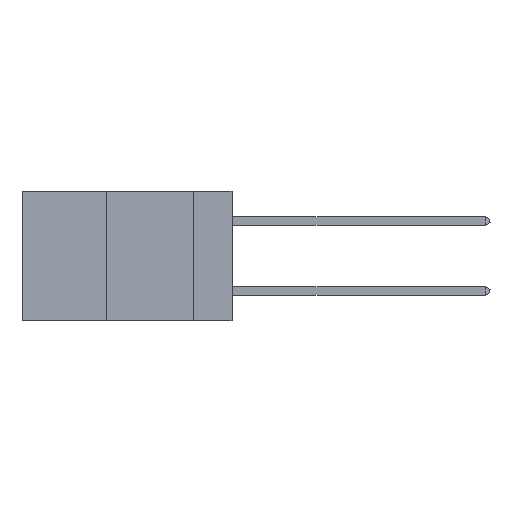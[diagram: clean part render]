
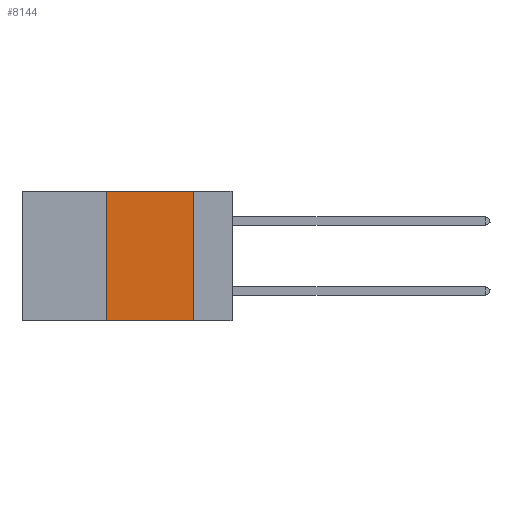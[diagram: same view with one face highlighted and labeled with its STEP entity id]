
A CAD part, left-side view. The second image highlights one B-rep face of the part: STEP entity #8144.
In plain terms, the highlighted planar face has unit normal (-1, 0, 0).
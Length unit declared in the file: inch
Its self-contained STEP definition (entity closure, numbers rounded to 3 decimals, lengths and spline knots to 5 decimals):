
#638 = LINE ( 'NONE', #2945, #24386 ) ;
#920 = ORIENTED_EDGE ( 'NONE', *, *, #11579, .F. ) ;
#1617 = CARTESIAN_POINT ( 'NONE',  ( 0., 0.6, 0. ) ) ;
#2262 = ORIENTED_EDGE ( 'NONE', *, *, #23073, .F. ) ;
#2395 = CARTESIAN_POINT ( 'NONE',  ( 0., 0.6, -0.37 ) ) ;
#2945 = CARTESIAN_POINT ( 'NONE',  ( 0., 0.36, 0. ) ) ;
#3497 = PLANE ( 'NONE',  #5939 ) ;
#3648 = VERTEX_POINT ( 'NONE', #21948 ) ;
#3904 = CARTESIAN_POINT ( 'NONE',  ( 0., 0.11, 0. ) ) ;
#4385 = DIRECTION ( 'NONE',  ( 0., -1., 0. ) ) ;
#5228 = DIRECTION ( 'NONE',  ( 0., 0., -1. ) ) ;
#5530 = VERTEX_POINT ( 'NONE', #22397 ) ;
#5887 = FACE_OUTER_BOUND ( 'NONE', #7418, .T. ) ;
#5899 = ORIENTED_EDGE ( 'NONE', *, *, #10131, .F. ) ;
#5939 = AXIS2_PLACEMENT_3D ( 'NONE', #1617, #23471, #5228 ) ;
#6279 = VERTEX_POINT ( 'NONE', #11103 ) ;
#6689 = DIRECTION ( 'NONE',  ( 0., 0., -1. ) ) ;
#7055 = LINE ( 'NONE', #20627, #19921 ) ;
#7418 = EDGE_LOOP ( 'NONE', ( #2262, #5899, #920, #25217 ) ) ;
#8144 = ADVANCED_FACE ( 'NONE', ( #5887 ), #3497, .F. ) ;
#9019 = DIRECTION ( 'NONE',  ( 0., 0., 1. ) ) ;
#10131 = EDGE_CURVE ( 'NONE', #5530, #15953, #14444, .T. ) ;
#10339 = LINE ( 'NONE', #2395, #24346 ) ;
#11103 = CARTESIAN_POINT ( 'NONE',  ( 0., 0.36, -0.37 ) ) ;
#11579 = EDGE_CURVE ( 'NONE', #6279, #5530, #638, .T. ) ;
#12869 = VECTOR ( 'NONE', #25792, 39.37008 ) ;
#14444 = LINE ( 'NONE', #17802, #12869 ) ;
#15953 = VERTEX_POINT ( 'NONE', #3904 ) ;
#15998 = EDGE_CURVE ( 'NONE', #6279, #3648, #10339, .T. ) ;
#17802 = CARTESIAN_POINT ( 'NONE',  ( 0., 0.6, 0. ) ) ;
#19921 = VECTOR ( 'NONE', #6689, 39.37008 ) ;
#20627 = CARTESIAN_POINT ( 'NONE',  ( 0., 0.11, 0. ) ) ;
#21948 = CARTESIAN_POINT ( 'NONE',  ( 0., 0.11, -0.37 ) ) ;
#22397 = CARTESIAN_POINT ( 'NONE',  ( 0., 0.36, 0. ) ) ;
#23073 = EDGE_CURVE ( 'NONE', #15953, #3648, #7055, .T. ) ;
#23471 = DIRECTION ( 'NONE',  ( 1., 0., 0. ) ) ;
#24346 = VECTOR ( 'NONE', #4385, 39.37008 ) ;
#24386 = VECTOR ( 'NONE', #9019, 39.37008 ) ;
#25217 = ORIENTED_EDGE ( 'NONE', *, *, #15998, .T. ) ;
#25792 = DIRECTION ( 'NONE',  ( 0., -1., 0. ) ) ;
